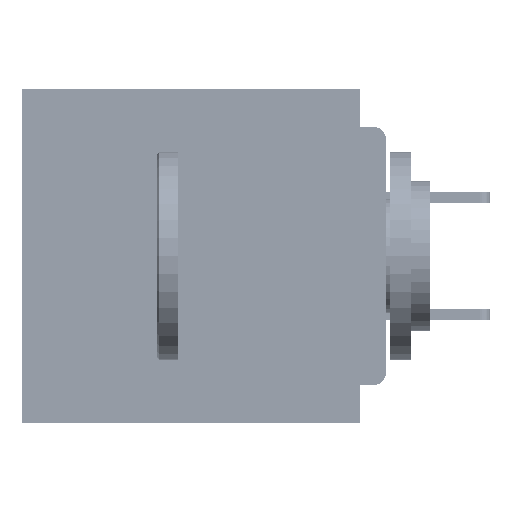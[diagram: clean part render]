
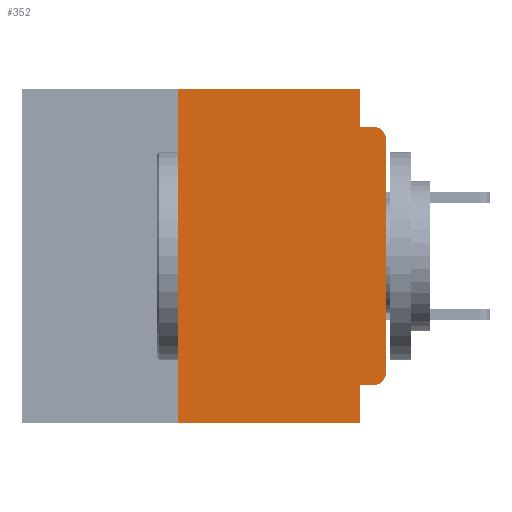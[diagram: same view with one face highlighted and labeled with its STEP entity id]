
A CAD part, left-side view. The second image highlights one B-rep face of the part: STEP entity #352.
In plain terms, the highlighted planar face has unit normal (-1, 0, 0).
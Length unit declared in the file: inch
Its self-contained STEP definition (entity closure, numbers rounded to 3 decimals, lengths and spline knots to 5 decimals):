
#352 = ADVANCED_FACE ( 'NONE', ( #11300 ), #59779, .F. ) ;
#1744 = CARTESIAN_POINT ( 'NONE',  ( 0., 0.437, 0. ) ) ;
#1879 = DIRECTION ( 'NONE',  ( 0., 0., 1. ) ) ;
#3694 = LINE ( 'NONE', #7418, #45861 ) ;
#3910 = ORIENTED_EDGE ( 'NONE', *, *, #52160, .F. ) ;
#5025 = ORIENTED_EDGE ( 'NONE', *, *, #24913, .T. ) ;
#5147 = CIRCLE ( 'NONE', #10299, 0.015 ) ;
#5558 = EDGE_CURVE ( 'NONE', #46579, #58298, #22923, .T. ) ;
#5651 = DIRECTION ( 'NONE',  ( -1., 0., 0. ) ) ;
#5942 = CARTESIAN_POINT ( 'NONE',  ( 0., 0.437, -0.4 ) ) ;
#5975 = VECTOR ( 'NONE', #60069, 39.37008 ) ;
#7011 = VERTEX_POINT ( 'NONE', #63054 ) ;
#7278 = DIRECTION ( 'NONE',  ( 0., -1., 0. ) ) ;
#7418 = CARTESIAN_POINT ( 'NONE',  ( 0., 0.25, -0.4 ) ) ;
#8643 = AXIS2_PLACEMENT_3D ( 'NONE', #38593, #5651, #44132 ) ;
#9956 = CARTESIAN_POINT ( 'NONE',  ( 0., 0.031, -0.4 ) ) ;
#10299 = AXIS2_PLACEMENT_3D ( 'NONE', #47133, #14202, #52670 ) ;
#10937 = EDGE_CURVE ( 'NONE', #7011, #29860, #50119, .T. ) ;
#11300 = FACE_OUTER_BOUND ( 'NONE', #20907, .T. ) ;
#11327 = ORIENTED_EDGE ( 'NONE', *, *, #26533, .T. ) ;
#11504 = DIRECTION ( 'NONE',  ( 0., -1., 0. ) ) ;
#12366 = CARTESIAN_POINT ( 'NONE',  ( 0., 0.25, -0.4 ) ) ;
#14202 = DIRECTION ( 'NONE',  ( -1., 0., 0. ) ) ;
#14789 = CIRCLE ( 'NONE', #8643, 0.015 ) ;
#16863 = VERTEX_POINT ( 'NONE', #28401 ) ;
#18551 = ORIENTED_EDGE ( 'NONE', *, *, #23973, .F. ) ;
#18650 = ORIENTED_EDGE ( 'NONE', *, *, #5558, .F. ) ;
#19484 = VECTOR ( 'NONE', #48176, 39.37008 ) ;
#20155 = CARTESIAN_POINT ( 'NONE',  ( 0., 0.25, 0. ) ) ;
#20843 = CARTESIAN_POINT ( 'NONE',  ( 0., 0., -0.06 ) ) ;
#20907 = EDGE_LOOP ( 'NONE', ( #29607, #5025, #3910, #35077, #71289, #18551, #11327, #18650, #62139, #65268 ) ) ;
#22923 = LINE ( 'NONE', #58977, #19484 ) ;
#23129 = VECTOR ( 'NONE', #11504, 39.37008 ) ;
#23973 = EDGE_CURVE ( 'NONE', #61374, #31379, #3694, .T. ) ;
#24597 = EDGE_CURVE ( 'NONE', #60389, #50734, #33761, .T. ) ;
#24913 = EDGE_CURVE ( 'NONE', #50734, #16863, #14789, .T. ) ;
#26130 = CARTESIAN_POINT ( 'NONE',  ( 0., 0.031, 0. ) ) ;
#26533 = EDGE_CURVE ( 'NONE', #61374, #58298, #67037, .T. ) ;
#28401 = CARTESIAN_POINT ( 'NONE',  ( 0., 0.015, -0.045 ) ) ;
#29225 = AXIS2_PLACEMENT_3D ( 'NONE', #59705, #70536, #70693 ) ;
#29607 = ORIENTED_EDGE ( 'NONE', *, *, #24597, .T. ) ;
#29860 = VERTEX_POINT ( 'NONE', #34526 ) ;
#31379 = VERTEX_POINT ( 'NONE', #20155 ) ;
#33761 = LINE ( 'NONE', #35978, #61285 ) ;
#34526 = CARTESIAN_POINT ( 'NONE',  ( 0., 0.031, -0.045 ) ) ;
#35077 = ORIENTED_EDGE ( 'NONE', *, *, #10937, .F. ) ;
#35223 = LINE ( 'NONE', #65859, #5975 ) ;
#35289 = LINE ( 'NONE', #1744, #62790 ) ;
#35978 = CARTESIAN_POINT ( 'NONE',  ( 0., 0., 0. ) ) ;
#38274 = CARTESIAN_POINT ( 'NONE',  ( 0., 0., -0.34 ) ) ;
#38593 = CARTESIAN_POINT ( 'NONE',  ( 0., 0.015, -0.06 ) ) ;
#39097 = VERTEX_POINT ( 'NONE', #43320 ) ;
#42471 = DIRECTION ( 'NONE',  ( 0., 0., -1. ) ) ;
#42857 = VECTOR ( 'NONE', #50972, 39.37008 ) ;
#43320 = CARTESIAN_POINT ( 'NONE',  ( 0., 0.015, -0.355 ) ) ;
#44132 = DIRECTION ( 'NONE',  ( 0., 0., -1. ) ) ;
#45861 = VECTOR ( 'NONE', #1879, 39.37008 ) ;
#46579 = VERTEX_POINT ( 'NONE', #62812 ) ;
#47133 = CARTESIAN_POINT ( 'NONE',  ( 0., 0.015, -0.34 ) ) ;
#48176 = DIRECTION ( 'NONE',  ( 0., 0., -1. ) ) ;
#50119 = LINE ( 'NONE', #26130, #64772 ) ;
#50734 = VERTEX_POINT ( 'NONE', #20843 ) ;
#50972 = DIRECTION ( 'NONE',  ( 0., 1., 0. ) ) ;
#51106 = EDGE_CURVE ( 'NONE', #31379, #7011, #35289, .T. ) ;
#52160 = EDGE_CURVE ( 'NONE', #29860, #16863, #35223, .T. ) ;
#52670 = DIRECTION ( 'NONE',  ( 0., 0., -1. ) ) ;
#56275 = CARTESIAN_POINT ( 'NONE',  ( 0., 0., -0.355 ) ) ;
#58298 = VERTEX_POINT ( 'NONE', #9956 ) ;
#58977 = CARTESIAN_POINT ( 'NONE',  ( 0., 0.031, -0.4 ) ) ;
#59705 = CARTESIAN_POINT ( 'NONE',  ( 0., 0.437, 0. ) ) ;
#59779 = PLANE ( 'NONE',  #29225 ) ;
#60069 = DIRECTION ( 'NONE',  ( 0., -1., 0. ) ) ;
#60389 = VERTEX_POINT ( 'NONE', #38274 ) ;
#60556 = EDGE_CURVE ( 'NONE', #39097, #46579, #60942, .T. ) ;
#60942 = LINE ( 'NONE', #56275, #42857 ) ;
#61285 = VECTOR ( 'NONE', #68956, 39.37008 ) ;
#61374 = VERTEX_POINT ( 'NONE', #12366 ) ;
#62139 = ORIENTED_EDGE ( 'NONE', *, *, #60556, .F. ) ;
#62790 = VECTOR ( 'NONE', #7278, 39.37008 ) ;
#62812 = CARTESIAN_POINT ( 'NONE',  ( 0., 0.031, -0.355 ) ) ;
#63054 = CARTESIAN_POINT ( 'NONE',  ( 0., 0.031, 0. ) ) ;
#63992 = EDGE_CURVE ( 'NONE', #39097, #60389, #5147, .T. ) ;
#64772 = VECTOR ( 'NONE', #42471, 39.37008 ) ;
#65268 = ORIENTED_EDGE ( 'NONE', *, *, #63992, .T. ) ;
#65859 = CARTESIAN_POINT ( 'NONE',  ( 0., 0., -0.045 ) ) ;
#67037 = LINE ( 'NONE', #5942, #23129 ) ;
#68956 = DIRECTION ( 'NONE',  ( 0., 0., 1. ) ) ;
#70536 = DIRECTION ( 'NONE',  ( 1., 0., 0. ) ) ;
#70693 = DIRECTION ( 'NONE',  ( 0., 0., -1. ) ) ;
#71289 = ORIENTED_EDGE ( 'NONE', *, *, #51106, .F. ) ;
